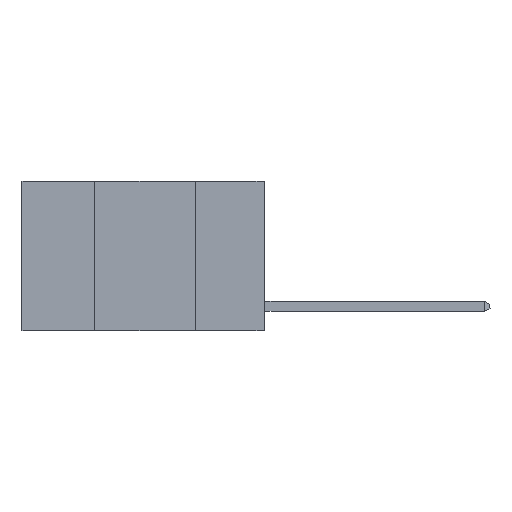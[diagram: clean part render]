
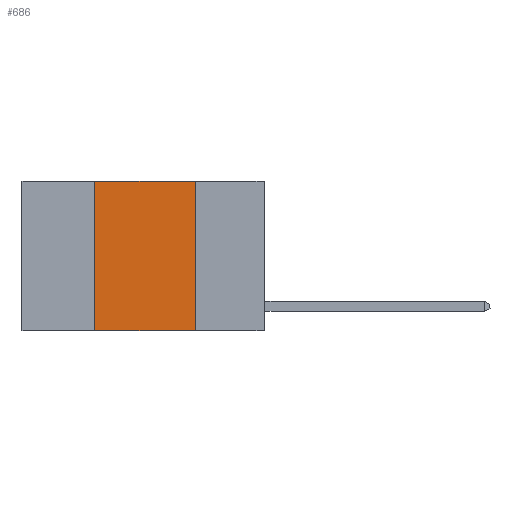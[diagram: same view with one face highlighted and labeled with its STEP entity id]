
A CAD part, left-side view. The second image highlights one B-rep face of the part: STEP entity #686.
In plain terms, the highlighted planar face has unit normal (-1, 0, 0).
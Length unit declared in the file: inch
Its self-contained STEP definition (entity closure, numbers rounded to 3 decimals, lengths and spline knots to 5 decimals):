
#175 = LINE ( 'NONE', #7319, #1867 ) ;
#580 = ORIENTED_EDGE ( 'NONE', *, *, #5681, .F. ) ;
#623 = CARTESIAN_POINT ( 'NONE',  ( 0., 0.42, 0. ) ) ;
#686 = ADVANCED_FACE ( 'NONE', ( #4868 ), #4168, .F. ) ;
#779 = CARTESIAN_POINT ( 'NONE',  ( 0., 0.6, 0. ) ) ;
#1025 = EDGE_LOOP ( 'NONE', ( #3242, #580, #1889, #9040 ) ) ;
#1323 = CARTESIAN_POINT ( 'NONE',  ( 0., 0.6, 0. ) ) ;
#1867 = VECTOR ( 'NONE', #8676, 39.37008 ) ;
#1889 = ORIENTED_EDGE ( 'NONE', *, *, #6841, .F. ) ;
#1928 = CARTESIAN_POINT ( 'NONE',  ( 0., 0.42, 0. ) ) ;
#2476 = AXIS2_PLACEMENT_3D ( 'NONE', #1323, #3448, #4352 ) ;
#2561 = VERTEX_POINT ( 'NONE', #623 ) ;
#2956 = DIRECTION ( 'NONE',  ( 0., -1., 0. ) ) ;
#3236 = CARTESIAN_POINT ( 'NONE',  ( 0., 0.42, -0.37 ) ) ;
#3242 = ORIENTED_EDGE ( 'NONE', *, *, #7028, .F. ) ;
#3448 = DIRECTION ( 'NONE',  ( 1., 0., 0. ) ) ;
#3948 = LINE ( 'NONE', #1928, #4526 ) ;
#4168 = PLANE ( 'NONE',  #2476 ) ;
#4352 = DIRECTION ( 'NONE',  ( 0., 0., -1. ) ) ;
#4526 = VECTOR ( 'NONE', #8997, 39.37008 ) ;
#4646 = DIRECTION ( 'NONE',  ( 0., -1., 0. ) ) ;
#4868 = FACE_OUTER_BOUND ( 'NONE', #1025, .T. ) ;
#4908 = VERTEX_POINT ( 'NONE', #8664 ) ;
#5205 = VERTEX_POINT ( 'NONE', #3236 ) ;
#5287 = EDGE_CURVE ( 'NONE', #5205, #7139, #7907, .T. ) ;
#5681 = EDGE_CURVE ( 'NONE', #2561, #4908, #7143, .T. ) ;
#5759 = CARTESIAN_POINT ( 'NONE',  ( 0., 0.6, -0.37 ) ) ;
#6575 = VECTOR ( 'NONE', #4646, 39.37008 ) ;
#6841 = EDGE_CURVE ( 'NONE', #5205, #2561, #3948, .T. ) ;
#7028 = EDGE_CURVE ( 'NONE', #4908, #7139, #175, .T. ) ;
#7139 = VERTEX_POINT ( 'NONE', #8630 ) ;
#7143 = LINE ( 'NONE', #779, #6575 ) ;
#7319 = CARTESIAN_POINT ( 'NONE',  ( 0., 0.17, 0. ) ) ;
#7907 = LINE ( 'NONE', #5759, #8542 ) ;
#8542 = VECTOR ( 'NONE', #2956, 39.37008 ) ;
#8630 = CARTESIAN_POINT ( 'NONE',  ( 0., 0.17, -0.37 ) ) ;
#8664 = CARTESIAN_POINT ( 'NONE',  ( 0., 0.17, 0. ) ) ;
#8676 = DIRECTION ( 'NONE',  ( 0., 0., -1. ) ) ;
#8997 = DIRECTION ( 'NONE',  ( 0., 0., 1. ) ) ;
#9040 = ORIENTED_EDGE ( 'NONE', *, *, #5287, .T. ) ;
